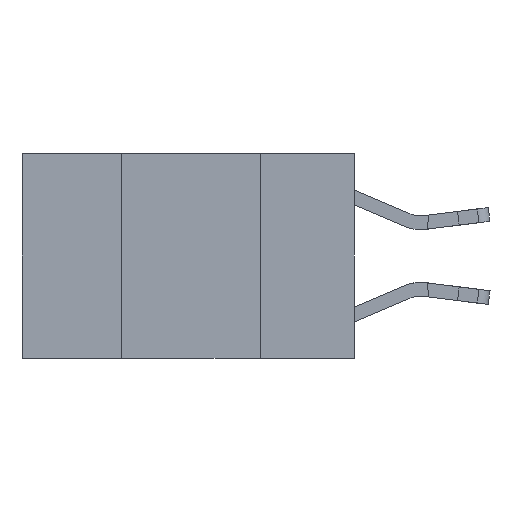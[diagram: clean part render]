
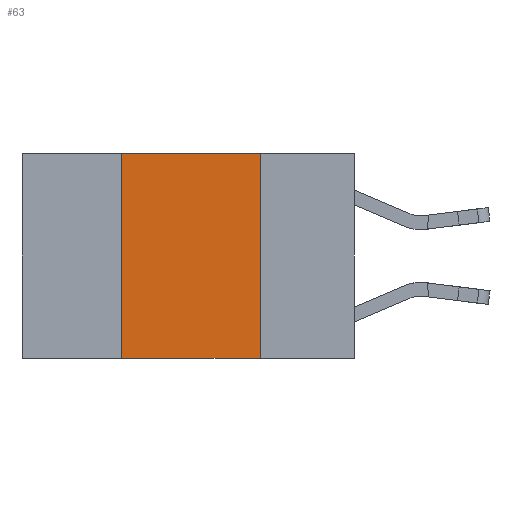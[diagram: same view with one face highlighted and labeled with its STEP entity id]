
A CAD part, left-side view. The second image highlights one B-rep face of the part: STEP entity #63.
In plain terms, the highlighted planar face has unit normal (-1, 0, 0).
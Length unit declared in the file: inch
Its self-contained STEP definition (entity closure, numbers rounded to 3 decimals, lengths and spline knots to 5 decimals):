
#63 = ADVANCED_FACE ( 'NONE', ( #4537 ), #3739, .F. ) ;
#527 = VERTEX_POINT ( 'NONE', #2888 ) ;
#622 = VECTOR ( 'NONE', #8950, 39.37008 ) ;
#799 = ORIENTED_EDGE ( 'NONE', *, *, #9472, .T. ) ;
#920 = CARTESIAN_POINT ( 'NONE',  ( 0., 0.42, 0. ) ) ;
#973 = EDGE_LOOP ( 'NONE', ( #1205, #4397, #3630, #799 ) ) ;
#1205 = ORIENTED_EDGE ( 'NONE', *, *, #9405, .F. ) ;
#1309 = DIRECTION ( 'NONE',  ( 0., 0., -1. ) ) ;
#1828 = VERTEX_POINT ( 'NONE', #3521 ) ;
#2154 = LINE ( 'NONE', #14820, #5356 ) ;
#2214 = VECTOR ( 'NONE', #5752, 39.37008 ) ;
#2481 = EDGE_CURVE ( 'NONE', #1828, #527, #3824, .T. ) ;
#2597 = LINE ( 'NONE', #920, #2214 ) ;
#2869 = CARTESIAN_POINT ( 'NONE',  ( 0., 0.42, -0.37 ) ) ;
#2888 = CARTESIAN_POINT ( 'NONE',  ( 0., 0.17, 0. ) ) ;
#3521 = CARTESIAN_POINT ( 'NONE',  ( 0., 0.42, 0. ) ) ;
#3630 = ORIENTED_EDGE ( 'NONE', *, *, #7681, .F. ) ;
#3731 = VERTEX_POINT ( 'NONE', #2869 ) ;
#3739 = PLANE ( 'NONE',  #14279 ) ;
#3824 = LINE ( 'NONE', #9041, #622 ) ;
#4397 = ORIENTED_EDGE ( 'NONE', *, *, #2481, .F. ) ;
#4537 = FACE_OUTER_BOUND ( 'NONE', #973, .T. ) ;
#5223 = CARTESIAN_POINT ( 'NONE',  ( 0., 0.17, 0. ) ) ;
#5356 = VECTOR ( 'NONE', #10051, 39.37008 ) ;
#5752 = DIRECTION ( 'NONE',  ( 0., 0., 1. ) ) ;
#7158 = VERTEX_POINT ( 'NONE', #9583 ) ;
#7681 = EDGE_CURVE ( 'NONE', #3731, #1828, #2597, .T. ) ;
#8950 = DIRECTION ( 'NONE',  ( 0., -1., 0. ) ) ;
#9041 = CARTESIAN_POINT ( 'NONE',  ( 0., 0.6, 0. ) ) ;
#9238 = LINE ( 'NONE', #5223, #12791 ) ;
#9405 = EDGE_CURVE ( 'NONE', #527, #7158, #9238, .T. ) ;
#9472 = EDGE_CURVE ( 'NONE', #3731, #7158, #2154, .T. ) ;
#9583 = CARTESIAN_POINT ( 'NONE',  ( 0., 0.17, -0.37 ) ) ;
#10051 = DIRECTION ( 'NONE',  ( 0., -1., 0. ) ) ;
#12292 = CARTESIAN_POINT ( 'NONE',  ( 0., 0.6, 0. ) ) ;
#12791 = VECTOR ( 'NONE', #14717, 39.37008 ) ;
#14279 = AXIS2_PLACEMENT_3D ( 'NONE', #12292, #15436, #1309 ) ;
#14717 = DIRECTION ( 'NONE',  ( 0., 0., -1. ) ) ;
#14820 = CARTESIAN_POINT ( 'NONE',  ( 0., 0.6, -0.37 ) ) ;
#15436 = DIRECTION ( 'NONE',  ( 1., 0., 0. ) ) ;
